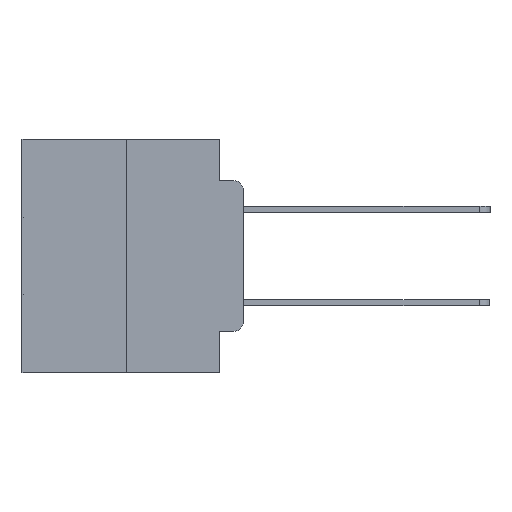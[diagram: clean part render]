
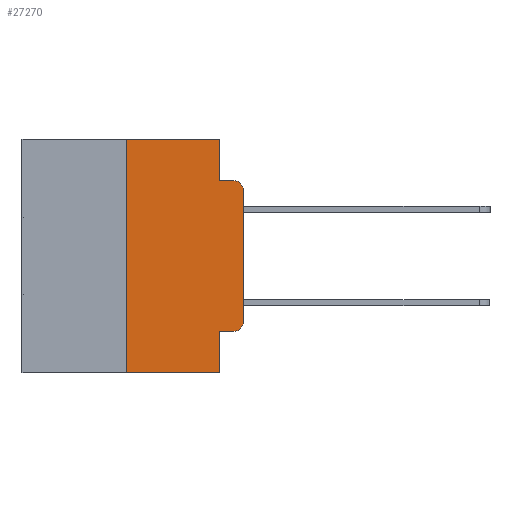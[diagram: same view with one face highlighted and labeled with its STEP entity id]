
A CAD part, left-side view. The second image highlights one B-rep face of the part: STEP entity #27270.
In plain terms, the highlighted planar face has unit normal (-1, 0, 0).
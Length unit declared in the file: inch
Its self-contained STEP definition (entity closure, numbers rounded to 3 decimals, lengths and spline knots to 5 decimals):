
#256 = EDGE_CURVE ( 'NONE', #10198, #348, #24876, .T. ) ;
#348 = VERTEX_POINT ( 'NONE', #24943 ) ;
#542 = EDGE_LOOP ( 'NONE', ( #26329, #25141, #25072, #4159, #17608, #15483, #14939, #22545, #17800, #18597 ) ) ;
#965 = VECTOR ( 'NONE', #4842, 39.37008 ) ;
#2118 = DIRECTION ( 'NONE',  ( 0., -1., 0. ) ) ;
#2291 = VECTOR ( 'NONE', #9286, 39.37008 ) ;
#2541 = VERTEX_POINT ( 'NONE', #16025 ) ;
#3031 = LINE ( 'NONE', #23431, #8297 ) ;
#3292 = DIRECTION ( 'NONE',  ( -1., 0., 0. ) ) ;
#3359 = DIRECTION ( 'NONE',  ( 0., -1., 0. ) ) ;
#4023 = CARTESIAN_POINT ( 'NONE',  ( 0., 0.25, 0. ) ) ;
#4159 = ORIENTED_EDGE ( 'NONE', *, *, #4790, .F. ) ;
#4397 = EDGE_CURVE ( 'NONE', #14934, #10195, #15492, .T. ) ;
#4453 = CARTESIAN_POINT ( 'NONE',  ( 0., 0.473, 0. ) ) ;
#4554 = PLANE ( 'NONE',  #13211 ) ;
#4790 = EDGE_CURVE ( 'NONE', #8015, #12217, #11702, .T. ) ;
#4842 = DIRECTION ( 'NONE',  ( 0., 0., -1. ) ) ;
#4912 = VERTEX_POINT ( 'NONE', #20054 ) ;
#5462 = VECTOR ( 'NONE', #3359, 39.37008 ) ;
#6412 = DIRECTION ( 'NONE',  ( 0., 0., -1. ) ) ;
#6804 = DIRECTION ( 'NONE',  ( 1., 0., 0. ) ) ;
#6970 = DIRECTION ( 'NONE',  ( 0., -1., 0. ) ) ;
#8015 = VERTEX_POINT ( 'NONE', #19228 ) ;
#8297 = VECTOR ( 'NONE', #21141, 39.37008 ) ;
#8679 = CARTESIAN_POINT ( 'NONE',  ( 0., 0.02, -0.0885 ) ) ;
#9015 = VECTOR ( 'NONE', #2118, 39.37008 ) ;
#9060 = FACE_OUTER_BOUND ( 'NONE', #542, .T. ) ;
#9241 = CIRCLE ( 'NONE', #14074, 0.02 ) ;
#9286 = DIRECTION ( 'NONE',  ( 0., 0., 1. ) ) ;
#10195 = VERTEX_POINT ( 'NONE', #10877 ) ;
#10198 = VERTEX_POINT ( 'NONE', #28250 ) ;
#10877 = CARTESIAN_POINT ( 'NONE',  ( 0., 0., -0.1085 ) ) ;
#11365 = EDGE_CURVE ( 'NONE', #28370, #2541, #3031, .T. ) ;
#11702 = LINE ( 'NONE', #26168, #27020 ) ;
#11873 = EDGE_CURVE ( 'NONE', #12217, #20557, #12086, .T. ) ;
#12086 = LINE ( 'NONE', #21009, #5462 ) ;
#12217 = VERTEX_POINT ( 'NONE', #16201 ) ;
#12625 = EDGE_CURVE ( 'NONE', #4912, #8015, #14876, .T. ) ;
#13211 = AXIS2_PLACEMENT_3D ( 'NONE', #4453, #6804, #22169 ) ;
#13236 = CARTESIAN_POINT ( 'NONE',  ( 0., 0.02, -0.3915 ) ) ;
#13301 = VECTOR ( 'NONE', #6970, 39.37008 ) ;
#13546 = LINE ( 'NONE', #24556, #965 ) ;
#13732 = EDGE_CURVE ( 'NONE', #28370, #4912, #16901, .T. ) ;
#14074 = AXIS2_PLACEMENT_3D ( 'NONE', #13236, #28382, #15423 ) ;
#14876 = LINE ( 'NONE', #19777, #9015 ) ;
#14934 = VERTEX_POINT ( 'NONE', #18384 ) ;
#14939 = ORIENTED_EDGE ( 'NONE', *, *, #11365, .T. ) ;
#15359 = EDGE_CURVE ( 'NONE', #348, #14934, #9241, .T. ) ;
#15423 = DIRECTION ( 'NONE',  ( 0., 0., -1. ) ) ;
#15483 = ORIENTED_EDGE ( 'NONE', *, *, #13732, .F. ) ;
#15492 = LINE ( 'NONE', #22377, #2291 ) ;
#16025 = CARTESIAN_POINT ( 'NONE',  ( 0., 0.051, -0.5 ) ) ;
#16201 = CARTESIAN_POINT ( 'NONE',  ( 0., 0.051, -0.0885 ) ) ;
#16564 = CARTESIAN_POINT ( 'NONE',  ( 0., 0.02, -0.1085 ) ) ;
#16901 = LINE ( 'NONE', #4023, #22659 ) ;
#17608 = ORIENTED_EDGE ( 'NONE', *, *, #12625, .F. ) ;
#17800 = ORIENTED_EDGE ( 'NONE', *, *, #256, .T. ) ;
#18378 = CARTESIAN_POINT ( 'NONE',  ( 0., 0.051, -0.4115 ) ) ;
#18384 = CARTESIAN_POINT ( 'NONE',  ( 0., 0., -0.3915 ) ) ;
#18597 = ORIENTED_EDGE ( 'NONE', *, *, #15359, .T. ) ;
#18745 = DIRECTION ( 'NONE',  ( 0., 0., -1. ) ) ;
#19228 = CARTESIAN_POINT ( 'NONE',  ( 0., 0.051, 0. ) ) ;
#19777 = CARTESIAN_POINT ( 'NONE',  ( 0., 0.473, 0. ) ) ;
#20054 = CARTESIAN_POINT ( 'NONE',  ( 0., 0.25, 0. ) ) ;
#20141 = CIRCLE ( 'NONE', #26577, 0.02 ) ;
#20557 = VERTEX_POINT ( 'NONE', #8679 ) ;
#21009 = CARTESIAN_POINT ( 'NONE',  ( 0., 0.051, -0.0885 ) ) ;
#21141 = DIRECTION ( 'NONE',  ( 0., -1., 0. ) ) ;
#21571 = EDGE_CURVE ( 'NONE', #10195, #20557, #20141, .T. ) ;
#22169 = DIRECTION ( 'NONE',  ( 0., 0., -1. ) ) ;
#22377 = CARTESIAN_POINT ( 'NONE',  ( 0., 0., 0. ) ) ;
#22545 = ORIENTED_EDGE ( 'NONE', *, *, #27375, .F. ) ;
#22659 = VECTOR ( 'NONE', #28146, 39.37008 ) ;
#23431 = CARTESIAN_POINT ( 'NONE',  ( 0., 0.473, -0.5 ) ) ;
#23638 = CARTESIAN_POINT ( 'NONE',  ( 0., 0.25, -0.5 ) ) ;
#24556 = CARTESIAN_POINT ( 'NONE',  ( 0., 0.051, 0. ) ) ;
#24876 = LINE ( 'NONE', #18378, #13301 ) ;
#24943 = CARTESIAN_POINT ( 'NONE',  ( 0., 0.02, -0.4115 ) ) ;
#25072 = ORIENTED_EDGE ( 'NONE', *, *, #11873, .F. ) ;
#25141 = ORIENTED_EDGE ( 'NONE', *, *, #21571, .T. ) ;
#26168 = CARTESIAN_POINT ( 'NONE',  ( 0., 0.051, 0. ) ) ;
#26329 = ORIENTED_EDGE ( 'NONE', *, *, #4397, .T. ) ;
#26577 = AXIS2_PLACEMENT_3D ( 'NONE', #16564, #3292, #18745 ) ;
#27020 = VECTOR ( 'NONE', #6412, 39.37008 ) ;
#27270 = ADVANCED_FACE ( 'NONE', ( #9060 ), #4554, .F. ) ;
#27375 = EDGE_CURVE ( 'NONE', #10198, #2541, #13546, .T. ) ;
#28146 = DIRECTION ( 'NONE',  ( 0., 0., 1. ) ) ;
#28250 = CARTESIAN_POINT ( 'NONE',  ( 0., 0.051, -0.4115 ) ) ;
#28370 = VERTEX_POINT ( 'NONE', #23638 ) ;
#28382 = DIRECTION ( 'NONE',  ( -1., 0., 0. ) ) ;
